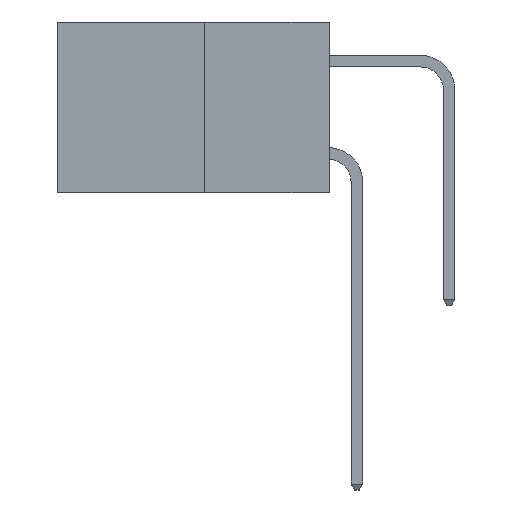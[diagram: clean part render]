
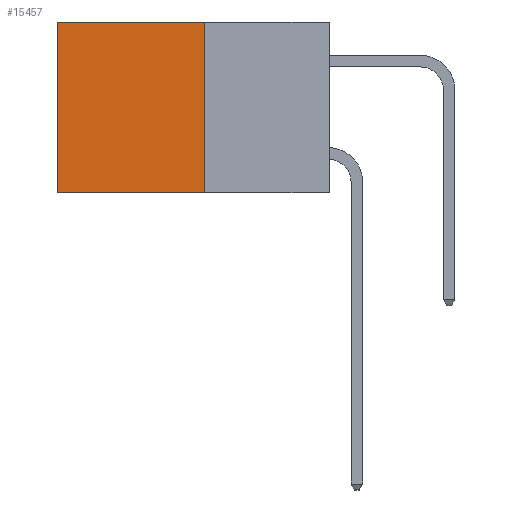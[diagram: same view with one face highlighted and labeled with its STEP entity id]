
A CAD part, left-side view. The second image highlights one B-rep face of the part: STEP entity #15457.
In plain terms, the highlighted planar face has unit normal (-1, 0, 0).
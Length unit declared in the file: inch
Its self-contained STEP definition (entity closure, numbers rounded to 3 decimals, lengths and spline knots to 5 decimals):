
#349 = LINE ( 'NONE', #12165, #6722 ) ;
#546 = PLANE ( 'NONE',  #1725 ) ;
#672 = VECTOR ( 'NONE', #3569, 39.37008 ) ;
#1025 = ORIENTED_EDGE ( 'NONE', *, *, #4865, .T. ) ;
#1195 = EDGE_CURVE ( 'NONE', #10122, #12552, #8303, .T. ) ;
#1725 = AXIS2_PLACEMENT_3D ( 'NONE', #1894, #11197, #3291 ) ;
#1894 = CARTESIAN_POINT ( 'NONE',  ( 0.277, 0.27, -0.37 ) ) ;
#1947 = CARTESIAN_POINT ( 'NONE',  ( 0.277, 0.27, -0.37 ) ) ;
#2407 = VERTEX_POINT ( 'NONE', #8371 ) ;
#2984 = CARTESIAN_POINT ( 'NONE',  ( 0.277, 0.27, -0.37 ) ) ;
#3291 = DIRECTION ( 'NONE',  ( 0., 0., -1. ) ) ;
#3569 = DIRECTION ( 'NONE',  ( 0., 0., -1. ) ) ;
#4200 = LINE ( 'NONE', #15772, #7353 ) ;
#4448 = ORIENTED_EDGE ( 'NONE', *, *, #6997, .T. ) ;
#4865 = EDGE_CURVE ( 'NONE', #10122, #2407, #4200, .T. ) ;
#6144 = ORIENTED_EDGE ( 'NONE', *, *, #8736, .F. ) ;
#6722 = VECTOR ( 'NONE', #12926, 39.37008 ) ;
#6997 = EDGE_CURVE ( 'NONE', #2407, #10794, #349, .T. ) ;
#7353 = VECTOR ( 'NONE', #15807, 39.37008 ) ;
#8303 = LINE ( 'NONE', #2984, #672 ) ;
#8371 = CARTESIAN_POINT ( 'NONE',  ( 0.277, 0.59, 0. ) ) ;
#8736 = EDGE_CURVE ( 'NONE', #12552, #10794, #10495, .T. ) ;
#10122 = VERTEX_POINT ( 'NONE', #15662 ) ;
#10435 = ORIENTED_EDGE ( 'NONE', *, *, #1195, .F. ) ;
#10495 = LINE ( 'NONE', #14831, #16435 ) ;
#10794 = VERTEX_POINT ( 'NONE', #15743 ) ;
#11197 = DIRECTION ( 'NONE',  ( 1., 0., 0. ) ) ;
#11655 = FACE_OUTER_BOUND ( 'NONE', #12565, .T. ) ;
#12165 = CARTESIAN_POINT ( 'NONE',  ( 0.277, 0.59, -0.37 ) ) ;
#12552 = VERTEX_POINT ( 'NONE', #1947 ) ;
#12565 = EDGE_LOOP ( 'NONE', ( #4448, #6144, #10435, #1025 ) ) ;
#12926 = DIRECTION ( 'NONE',  ( 0., 0., -1. ) ) ;
#14831 = CARTESIAN_POINT ( 'NONE',  ( 0.277, 0.27, -0.37 ) ) ;
#15457 = ADVANCED_FACE ( 'NONE', ( #11655 ), #546, .F. ) ;
#15662 = CARTESIAN_POINT ( 'NONE',  ( 0.277, 0.27, 0. ) ) ;
#15743 = CARTESIAN_POINT ( 'NONE',  ( 0.277, 0.59, -0.37 ) ) ;
#15772 = CARTESIAN_POINT ( 'NONE',  ( 0.277, 0.27, 0. ) ) ;
#15807 = DIRECTION ( 'NONE',  ( 0., 1., 0. ) ) ;
#15973 = DIRECTION ( 'NONE',  ( 0., 1., 0. ) ) ;
#16435 = VECTOR ( 'NONE', #15973, 39.37008 ) ;
